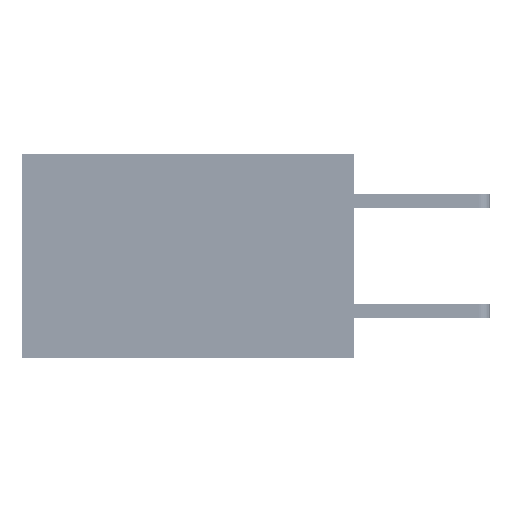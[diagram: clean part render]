
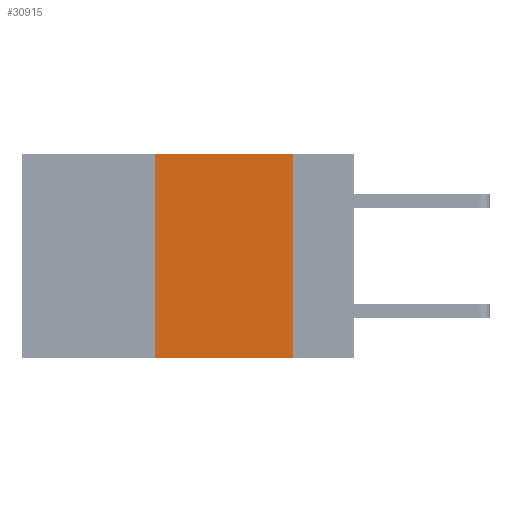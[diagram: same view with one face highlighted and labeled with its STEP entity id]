
A CAD part, left-side view. The second image highlights one B-rep face of the part: STEP entity #30915.
In plain terms, the highlighted planar face has unit normal (-1, 0, 0).
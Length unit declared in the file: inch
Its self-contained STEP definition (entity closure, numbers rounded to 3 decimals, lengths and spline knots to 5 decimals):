
#75 = EDGE_CURVE ( 'NONE', #35487, #30742, #17375, .T. ) ;
#530 = CARTESIAN_POINT ( 'NONE',  ( 0., 0.11, 0. ) ) ;
#1357 = CARTESIAN_POINT ( 'NONE',  ( 0., 0.36, 0. ) ) ;
#1647 = VERTEX_POINT ( 'NONE', #530 ) ;
#3522 = FACE_OUTER_BOUND ( 'NONE', #5010, .T. ) ;
#5010 = EDGE_LOOP ( 'NONE', ( #15370, #39506, #45988, #11996 ) ) ;
#5515 = LINE ( 'NONE', #12435, #12724 ) ;
#8397 = AXIS2_PLACEMENT_3D ( 'NONE', #27411, #32380, #23736 ) ;
#10850 = DIRECTION ( 'NONE',  ( 0., -1., 0. ) ) ;
#11504 = VECTOR ( 'NONE', #10850, 39.37008 ) ;
#11996 = ORIENTED_EDGE ( 'NONE', *, *, #32837, .T. ) ;
#12435 = CARTESIAN_POINT ( 'NONE',  ( 0., 0.6, -0.37 ) ) ;
#12724 = VECTOR ( 'NONE', #23988, 39.37008 ) ;
#15058 = LINE ( 'NONE', #30783, #11504 ) ;
#15120 = EDGE_CURVE ( 'NONE', #30742, #1647, #15058, .T. ) ;
#15370 = ORIENTED_EDGE ( 'NONE', *, *, #38146, .F. ) ;
#16843 = CARTESIAN_POINT ( 'NONE',  ( 0., 0.11, -0.37 ) ) ;
#17375 = LINE ( 'NONE', #1357, #29360 ) ;
#17862 = LINE ( 'NONE', #25715, #48760 ) ;
#23736 = DIRECTION ( 'NONE',  ( 0., 0., -1. ) ) ;
#23988 = DIRECTION ( 'NONE',  ( 0., -1., 0. ) ) ;
#25534 = DIRECTION ( 'NONE',  ( 0., 0., 1. ) ) ;
#25715 = CARTESIAN_POINT ( 'NONE',  ( 0., 0.11, 0. ) ) ;
#25928 = CARTESIAN_POINT ( 'NONE',  ( 0., 0.36, 0. ) ) ;
#27411 = CARTESIAN_POINT ( 'NONE',  ( 0., 0.6, 0. ) ) ;
#29360 = VECTOR ( 'NONE', #25534, 39.37008 ) ;
#30742 = VERTEX_POINT ( 'NONE', #25928 ) ;
#30783 = CARTESIAN_POINT ( 'NONE',  ( 0., 0.6, 0. ) ) ;
#30915 = ADVANCED_FACE ( 'NONE', ( #3522 ), #51595, .F. ) ;
#32380 = DIRECTION ( 'NONE',  ( 1., 0., 0. ) ) ;
#32837 = EDGE_CURVE ( 'NONE', #35487, #49603, #5515, .T. ) ;
#35487 = VERTEX_POINT ( 'NONE', #39319 ) ;
#38146 = EDGE_CURVE ( 'NONE', #1647, #49603, #17862, .T. ) ;
#39319 = CARTESIAN_POINT ( 'NONE',  ( 0., 0.36, -0.37 ) ) ;
#39506 = ORIENTED_EDGE ( 'NONE', *, *, #15120, .F. ) ;
#41727 = DIRECTION ( 'NONE',  ( 0., 0., -1. ) ) ;
#45988 = ORIENTED_EDGE ( 'NONE', *, *, #75, .F. ) ;
#48760 = VECTOR ( 'NONE', #41727, 39.37008 ) ;
#49603 = VERTEX_POINT ( 'NONE', #16843 ) ;
#51595 = PLANE ( 'NONE',  #8397 ) ;
